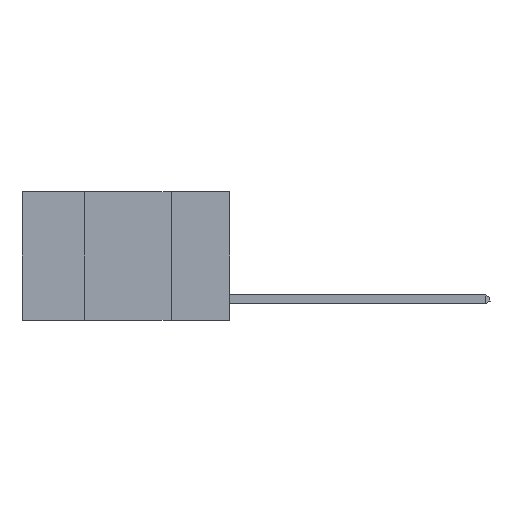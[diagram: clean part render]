
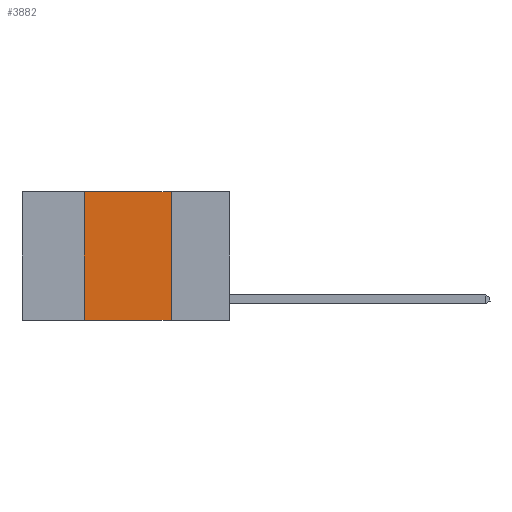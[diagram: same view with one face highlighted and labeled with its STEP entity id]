
A CAD part, left-side view. The second image highlights one B-rep face of the part: STEP entity #3882.
In plain terms, the highlighted planar face has unit normal (-1, 0, 0).
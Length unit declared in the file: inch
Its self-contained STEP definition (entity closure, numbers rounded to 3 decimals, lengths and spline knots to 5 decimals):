
#43 = EDGE_LOOP ( 'NONE', ( #3684, #16649, #9236, #392 ) ) ;
#392 = ORIENTED_EDGE ( 'NONE', *, *, #13303, .T. ) ;
#945 = LINE ( 'NONE', #10368, #3270 ) ;
#1040 = DIRECTION ( 'NONE',  ( 0., 0., 1. ) ) ;
#1849 = DIRECTION ( 'NONE',  ( 0., 0., -1. ) ) ;
#3089 = LINE ( 'NONE', #12621, #5558 ) ;
#3270 = VECTOR ( 'NONE', #1040, 39.37008 ) ;
#3279 = VECTOR ( 'NONE', #7549, 39.37008 ) ;
#3363 = VECTOR ( 'NONE', #4773, 39.37008 ) ;
#3564 = LINE ( 'NONE', #13275, #3279 ) ;
#3637 = DIRECTION ( 'NONE',  ( 1., 0., 0. ) ) ;
#3684 = ORIENTED_EDGE ( 'NONE', *, *, #4107, .F. ) ;
#3882 = ADVANCED_FACE ( 'NONE', ( #13340 ), #7779, .F. ) ;
#4107 = EDGE_CURVE ( 'NONE', #11878, #13901, #3089, .T. ) ;
#4773 = DIRECTION ( 'NONE',  ( 0., -1., 0. ) ) ;
#5558 = VECTOR ( 'NONE', #1849, 39.37008 ) ;
#6956 = AXIS2_PLACEMENT_3D ( 'NONE', #15634, #3637, #14378 ) ;
#7092 = VERTEX_POINT ( 'NONE', #16192 ) ;
#7549 = DIRECTION ( 'NONE',  ( 0., -1., 0. ) ) ;
#7550 = CARTESIAN_POINT ( 'NONE',  ( 0., 0.42, -0.37 ) ) ;
#7779 = PLANE ( 'NONE',  #6956 ) ;
#9236 = ORIENTED_EDGE ( 'NONE', *, *, #11668, .F. ) ;
#9277 = CARTESIAN_POINT ( 'NONE',  ( 0., 0.17, -0.37 ) ) ;
#10368 = CARTESIAN_POINT ( 'NONE',  ( 0., 0.42, 0. ) ) ;
#11668 = EDGE_CURVE ( 'NONE', #15498, #7092, #945, .T. ) ;
#11878 = VERTEX_POINT ( 'NONE', #16530 ) ;
#12621 = CARTESIAN_POINT ( 'NONE',  ( 0., 0.17, 0. ) ) ;
#13275 = CARTESIAN_POINT ( 'NONE',  ( 0., 0.6, -0.37 ) ) ;
#13303 = EDGE_CURVE ( 'NONE', #15498, #13901, #3564, .T. ) ;
#13340 = FACE_OUTER_BOUND ( 'NONE', #43, .T. ) ;
#13901 = VERTEX_POINT ( 'NONE', #9277 ) ;
#14210 = CARTESIAN_POINT ( 'NONE',  ( 0., 0.6, 0. ) ) ;
#14378 = DIRECTION ( 'NONE',  ( 0., 0., -1. ) ) ;
#15498 = VERTEX_POINT ( 'NONE', #7550 ) ;
#15634 = CARTESIAN_POINT ( 'NONE',  ( 0., 0.6, 0. ) ) ;
#16192 = CARTESIAN_POINT ( 'NONE',  ( 0., 0.42, 0. ) ) ;
#16530 = CARTESIAN_POINT ( 'NONE',  ( 0., 0.17, 0. ) ) ;
#16649 = ORIENTED_EDGE ( 'NONE', *, *, #17075, .F. ) ;
#17075 = EDGE_CURVE ( 'NONE', #7092, #11878, #17119, .T. ) ;
#17119 = LINE ( 'NONE', #14210, #3363 ) ;
